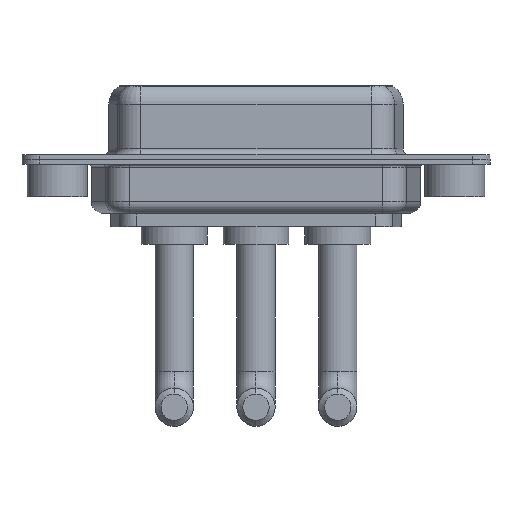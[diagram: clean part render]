
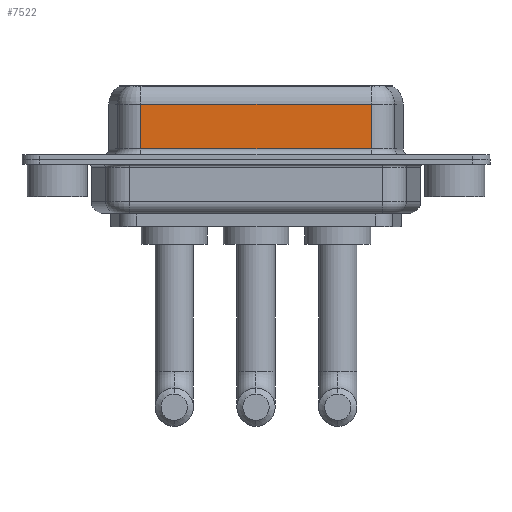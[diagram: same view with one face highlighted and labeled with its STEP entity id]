
A CAD part, front view. The second image highlights one B-rep face of the part: STEP entity #7522.
In plain terms, the highlighted planar face has unit normal (0, -1, 0).
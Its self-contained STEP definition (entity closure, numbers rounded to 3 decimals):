
#130 = VECTOR ( 'NONE', #6270, 1000. ) ;
#1245 = PLANE ( 'NONE',  #5572 ) ;
#1393 = VERTEX_POINT ( 'NONE', #5237 ) ;
#1978 = CARTESIAN_POINT ( 'NONE',  ( 26.287, -3.95, 6.4 ) ) ;
#2087 = VERTEX_POINT ( 'NONE', #11280 ) ;
#2184 = VERTEX_POINT ( 'NONE', #4914 ) ;
#2370 = CARTESIAN_POINT ( 'NONE',  ( 26.287, -3.95, 0.9 ) ) ;
#2407 = LINE ( 'NONE', #11761, #2877 ) ;
#2877 = VECTOR ( 'NONE', #6205, 1000. ) ;
#3110 = DIRECTION ( 'NONE',  ( 0., 0., 1. ) ) ;
#3170 = DIRECTION ( 'NONE',  ( 0., 1., 0. ) ) ;
#3459 = VERTEX_POINT ( 'NONE', #2370 ) ;
#4852 = ORIENTED_EDGE ( 'NONE', *, *, #10137, .T. ) ;
#4914 = CARTESIAN_POINT ( 'NONE',  ( 7.013, -3.95, 0.9 ) ) ;
#5034 = ORIENTED_EDGE ( 'NONE', *, *, #7138, .T. ) ;
#5237 = CARTESIAN_POINT ( 'NONE',  ( 26.287, -3.95, 4.65 ) ) ;
#5324 = ORIENTED_EDGE ( 'NONE', *, *, #7916, .T. ) ;
#5572 = AXIS2_PLACEMENT_3D ( 'NONE', #1978, #3170, #3110 ) ;
#6066 = EDGE_CURVE ( 'NONE', #1393, #3459, #11263, .T. ) ;
#6205 = DIRECTION ( 'NONE',  ( 1., 0., 0. ) ) ;
#6270 = DIRECTION ( 'NONE',  ( -1., 0., 0. ) ) ;
#6393 = CARTESIAN_POINT ( 'NONE',  ( 26.287, -3.95, 6.4 ) ) ;
#6457 = DIRECTION ( 'NONE',  ( 0., 0., -1. ) ) ;
#7090 = LINE ( 'NONE', #10127, #130 ) ;
#7138 = EDGE_CURVE ( 'NONE', #1393, #2087, #7090, .T. ) ;
#7522 = ADVANCED_FACE ( 'NONE', ( #11631 ), #1245, .F. ) ;
#7772 = LINE ( 'NONE', #8935, #8669 ) ;
#7886 = DIRECTION ( 'NONE',  ( 0., 0., -1. ) ) ;
#7916 = EDGE_CURVE ( 'NONE', #2087, #2184, #7772, .T. ) ;
#8669 = VECTOR ( 'NONE', #7886, 1000. ) ;
#8935 = CARTESIAN_POINT ( 'NONE',  ( 7.013, -3.95, 6.4 ) ) ;
#9649 = EDGE_LOOP ( 'NONE', ( #10839, #5034, #5324, #4852 ) ) ;
#10127 = CARTESIAN_POINT ( 'NONE',  ( 26.287, -3.95, 4.65 ) ) ;
#10137 = EDGE_CURVE ( 'NONE', #2184, #3459, #2407, .T. ) ;
#10326 = VECTOR ( 'NONE', #6457, 1000. ) ;
#10839 = ORIENTED_EDGE ( 'NONE', *, *, #6066, .F. ) ;
#11263 = LINE ( 'NONE', #6393, #10326 ) ;
#11280 = CARTESIAN_POINT ( 'NONE',  ( 7.013, -3.95, 4.65 ) ) ;
#11631 = FACE_OUTER_BOUND ( 'NONE', #9649, .T. ) ;
#11761 = CARTESIAN_POINT ( 'NONE',  ( 26.287, -3.95, 0.9 ) ) ;
